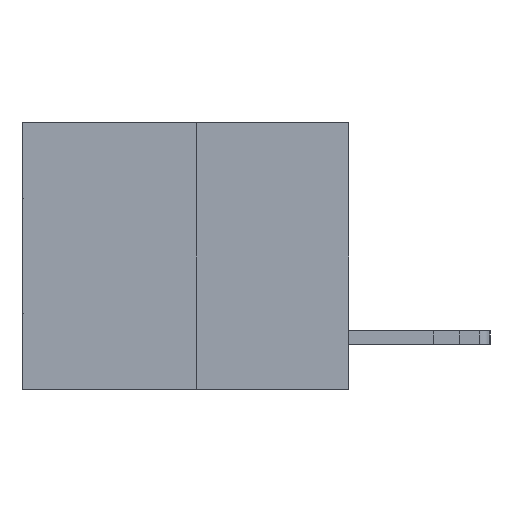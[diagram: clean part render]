
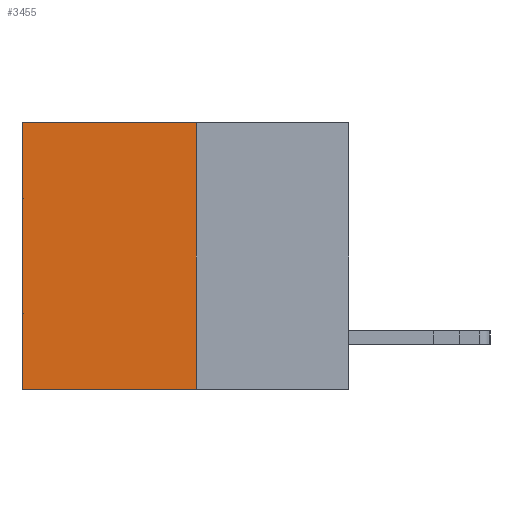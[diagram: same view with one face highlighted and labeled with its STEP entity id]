
A CAD part, left-side view. The second image highlights one B-rep face of the part: STEP entity #3455.
In plain terms, the highlighted planar face has unit normal (-1, 0, 0).
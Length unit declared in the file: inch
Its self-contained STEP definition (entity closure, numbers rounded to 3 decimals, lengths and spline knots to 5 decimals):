
#898 = LINE ( 'NONE', #1655, #27854 ) ;
#1655 = CARTESIAN_POINT ( 'NONE',  ( 0.3165, 0.6, -0.49 ) ) ;
#1827 = DIRECTION ( 'NONE',  ( 0., 0., -1. ) ) ;
#2783 = VECTOR ( 'NONE', #25764, 39.37008 ) ;
#3455 = ADVANCED_FACE ( 'NONE', ( #25112 ), #22544, .F. ) ;
#4076 = CARTESIAN_POINT ( 'NONE',  ( 0.3165, 0.28, 0. ) ) ;
#4096 = VERTEX_POINT ( 'NONE', #10047 ) ;
#4306 = VERTEX_POINT ( 'NONE', #17087 ) ;
#4867 = ORIENTED_EDGE ( 'NONE', *, *, #12499, .F. ) ;
#5606 = LINE ( 'NONE', #12339, #2783 ) ;
#6112 = EDGE_LOOP ( 'NONE', ( #17226, #4867, #21277, #14832 ) ) ;
#6642 = VECTOR ( 'NONE', #1827, 39.37008 ) ;
#7926 = DIRECTION ( 'NONE',  ( 0., 0., -1. ) ) ;
#8017 = LINE ( 'NONE', #17275, #6642 ) ;
#8628 = EDGE_CURVE ( 'NONE', #15286, #4306, #23708, .T. ) ;
#8810 = DIRECTION ( 'NONE',  ( 0., 0., -1. ) ) ;
#10047 = CARTESIAN_POINT ( 'NONE',  ( 0.3165, 0.28, -0.49 ) ) ;
#12339 = CARTESIAN_POINT ( 'NONE',  ( 0.3165, 0.28, -0.49 ) ) ;
#12499 = EDGE_CURVE ( 'NONE', #4096, #25557, #5606, .T. ) ;
#13237 = AXIS2_PLACEMENT_3D ( 'NONE', #13324, #20006, #8810 ) ;
#13324 = CARTESIAN_POINT ( 'NONE',  ( 0.3165, 0.28, -0.49 ) ) ;
#14097 = EDGE_CURVE ( 'NONE', #4306, #25557, #898, .T. ) ;
#14832 = ORIENTED_EDGE ( 'NONE', *, *, #8628, .T. ) ;
#15286 = VERTEX_POINT ( 'NONE', #4076 ) ;
#17087 = CARTESIAN_POINT ( 'NONE',  ( 0.3165, 0.6, 0. ) ) ;
#17226 = ORIENTED_EDGE ( 'NONE', *, *, #14097, .T. ) ;
#17275 = CARTESIAN_POINT ( 'NONE',  ( 0.3165, 0.28, -0.49 ) ) ;
#20006 = DIRECTION ( 'NONE',  ( 1., 0., 0. ) ) ;
#21277 = ORIENTED_EDGE ( 'NONE', *, *, #22904, .F. ) ;
#22544 = PLANE ( 'NONE',  #13237 ) ;
#22904 = EDGE_CURVE ( 'NONE', #15286, #4096, #8017, .T. ) ;
#23708 = LINE ( 'NONE', #26573, #25070 ) ;
#24855 = CARTESIAN_POINT ( 'NONE',  ( 0.3165, 0.6, -0.49 ) ) ;
#25070 = VECTOR ( 'NONE', #28505, 39.37008 ) ;
#25112 = FACE_OUTER_BOUND ( 'NONE', #6112, .T. ) ;
#25557 = VERTEX_POINT ( 'NONE', #24855 ) ;
#25764 = DIRECTION ( 'NONE',  ( 0., 1., 0. ) ) ;
#26573 = CARTESIAN_POINT ( 'NONE',  ( 0.3165, 0.28, 0. ) ) ;
#27854 = VECTOR ( 'NONE', #7926, 39.37008 ) ;
#28505 = DIRECTION ( 'NONE',  ( 0., 1., 0. ) ) ;
